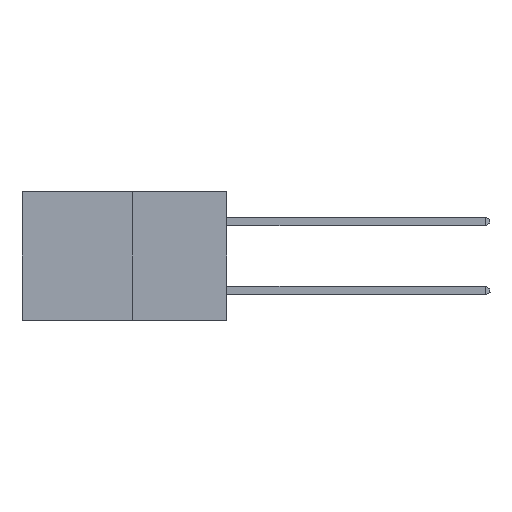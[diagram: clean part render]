
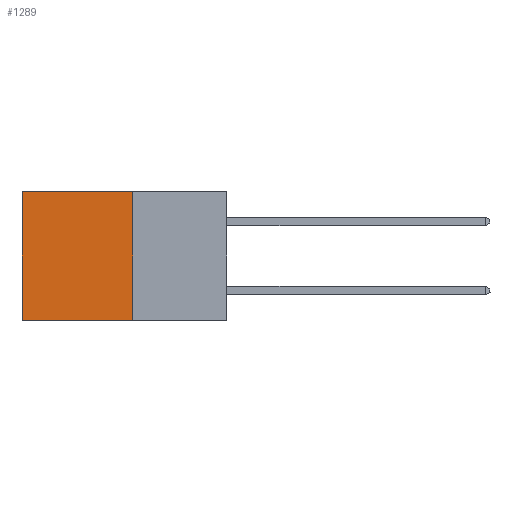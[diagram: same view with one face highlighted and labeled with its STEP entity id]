
A CAD part, left-side view. The second image highlights one B-rep face of the part: STEP entity #1289.
In plain terms, the highlighted planar face has unit normal (-1, 0, 0).
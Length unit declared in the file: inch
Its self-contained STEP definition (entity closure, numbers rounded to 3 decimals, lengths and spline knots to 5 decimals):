
#26 = ORIENTED_EDGE ( 'NONE', *, *, #11151, .T. ) ;
#310 = VECTOR ( 'NONE', #8725, 39.37008 ) ;
#772 = EDGE_CURVE ( 'NONE', #1445, #10202, #2791, .T. ) ;
#1289 = ADVANCED_FACE ( 'NONE', ( #8977 ), #6467, .F. ) ;
#1329 = ORIENTED_EDGE ( 'NONE', *, *, #3249, .F. ) ;
#1366 = ORIENTED_EDGE ( 'NONE', *, *, #10595, .T. ) ;
#1445 = VERTEX_POINT ( 'NONE', #5312 ) ;
#1824 = VERTEX_POINT ( 'NONE', #4745 ) ;
#2291 = ORIENTED_EDGE ( 'NONE', *, *, #772, .F. ) ;
#2368 = EDGE_LOOP ( 'NONE', ( #1366, #1329, #2291, #26 ) ) ;
#2791 = LINE ( 'NONE', #7635, #310 ) ;
#3163 = DIRECTION ( 'NONE',  ( 0., 0., -1. ) ) ;
#3249 = EDGE_CURVE ( 'NONE', #10202, #1824, #10210, .T. ) ;
#4275 = CARTESIAN_POINT ( 'NONE',  ( 0.277, 0.27, 0. ) ) ;
#4318 = VECTOR ( 'NONE', #11037, 39.37008 ) ;
#4745 = CARTESIAN_POINT ( 'NONE',  ( 0.277, 0.59, -0.37 ) ) ;
#5312 = CARTESIAN_POINT ( 'NONE',  ( 0.277, 0.27, 0. ) ) ;
#5351 = CARTESIAN_POINT ( 'NONE',  ( 0.277, 0.59, -0.37 ) ) ;
#5657 = CARTESIAN_POINT ( 'NONE',  ( 0.277, 0.27, -0.37 ) ) ;
#5772 = VECTOR ( 'NONE', #8254, 39.37008 ) ;
#6467 = PLANE ( 'NONE',  #7713 ) ;
#7474 = LINE ( 'NONE', #5351, #9905 ) ;
#7635 = CARTESIAN_POINT ( 'NONE',  ( 0.277, 0.27, -0.37 ) ) ;
#7713 = AXIS2_PLACEMENT_3D ( 'NONE', #8417, #10354, #3163 ) ;
#7758 = VERTEX_POINT ( 'NONE', #10670 ) ;
#8254 = DIRECTION ( 'NONE',  ( 0., 1., 0. ) ) ;
#8417 = CARTESIAN_POINT ( 'NONE',  ( 0.277, 0.27, -0.37 ) ) ;
#8667 = LINE ( 'NONE', #4275, #4318 ) ;
#8725 = DIRECTION ( 'NONE',  ( 0., 0., -1. ) ) ;
#8977 = FACE_OUTER_BOUND ( 'NONE', #2368, .T. ) ;
#9905 = VECTOR ( 'NONE', #11184, 39.37008 ) ;
#10202 = VERTEX_POINT ( 'NONE', #5657 ) ;
#10210 = LINE ( 'NONE', #10631, #5772 ) ;
#10354 = DIRECTION ( 'NONE',  ( 1., 0., 0. ) ) ;
#10595 = EDGE_CURVE ( 'NONE', #7758, #1824, #7474, .T. ) ;
#10631 = CARTESIAN_POINT ( 'NONE',  ( 0.277, 0.27, -0.37 ) ) ;
#10670 = CARTESIAN_POINT ( 'NONE',  ( 0.277, 0.59, 0. ) ) ;
#11037 = DIRECTION ( 'NONE',  ( 0., 1., 0. ) ) ;
#11151 = EDGE_CURVE ( 'NONE', #1445, #7758, #8667, .T. ) ;
#11184 = DIRECTION ( 'NONE',  ( 0., 0., -1. ) ) ;
